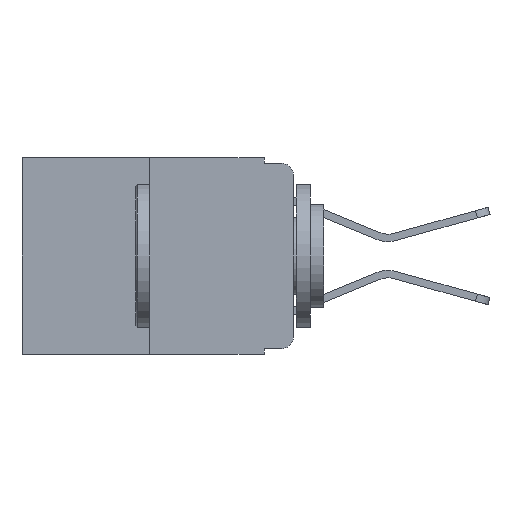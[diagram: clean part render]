
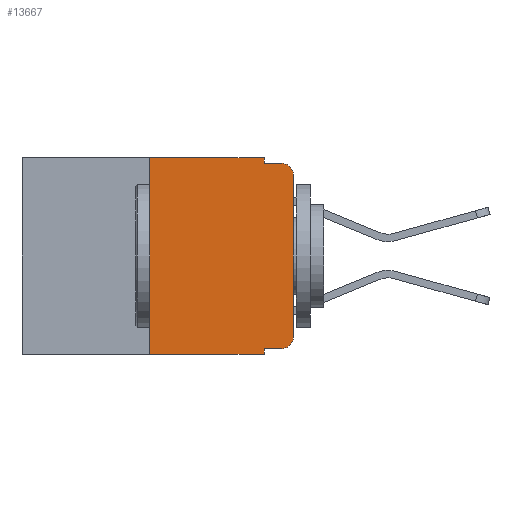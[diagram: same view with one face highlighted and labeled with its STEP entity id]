
A CAD part, left-side view. The second image highlights one B-rep face of the part: STEP entity #13667.
In plain terms, the highlighted planar face has unit normal (-1, 0, 0).
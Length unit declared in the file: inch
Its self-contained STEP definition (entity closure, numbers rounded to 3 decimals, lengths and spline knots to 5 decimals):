
#54 = VERTEX_POINT ( 'NONE', #13120 ) ;
#201 = DIRECTION ( 'NONE',  ( 0., 0., -1. ) ) ;
#498 = CARTESIAN_POINT ( 'NONE',  ( 0., 0.02, -0.333 ) ) ;
#555 = AXIS2_PLACEMENT_3D ( 'NONE', #2039, #13216, #3651 ) ;
#696 = CARTESIAN_POINT ( 'NONE',  ( 0., 0.051, 0. ) ) ;
#766 = CARTESIAN_POINT ( 'NONE',  ( 0., 0., -0.03 ) ) ;
#887 = DIRECTION ( 'NONE',  ( 0., 0., -1. ) ) ;
#2039 = CARTESIAN_POINT ( 'NONE',  ( 0., 0.473, 0. ) ) ;
#2335 = DIRECTION ( 'NONE',  ( 0., -1., 0. ) ) ;
#2366 = DIRECTION ( 'NONE',  ( 0., 0., -1. ) ) ;
#2546 = CARTESIAN_POINT ( 'NONE',  ( 0., 0.25, -0.343 ) ) ;
#2709 = CARTESIAN_POINT ( 'NONE',  ( 0., 0.473, 0. ) ) ;
#3063 = VECTOR ( 'NONE', #2366, 39.37008 ) ;
#3168 = VECTOR ( 'NONE', #6275, 39.37008 ) ;
#3325 = CARTESIAN_POINT ( 'NONE',  ( 0., 0.051, 0. ) ) ;
#3651 = DIRECTION ( 'NONE',  ( 0., 0., -1. ) ) ;
#3678 = ORIENTED_EDGE ( 'NONE', *, *, #8463, .T. ) ;
#3805 = VECTOR ( 'NONE', #9018, 39.37008 ) ;
#3898 = VERTEX_POINT ( 'NONE', #766 ) ;
#4137 = CIRCLE ( 'NONE', #9452, 0.02 ) ;
#4145 = VERTEX_POINT ( 'NONE', #18810 ) ;
#4224 = VERTEX_POINT ( 'NONE', #14356 ) ;
#4323 = LINE ( 'NONE', #2709, #3805 ) ;
#4458 = VERTEX_POINT ( 'NONE', #10040 ) ;
#5120 = VERTEX_POINT ( 'NONE', #498 ) ;
#5843 = EDGE_CURVE ( 'NONE', #19342, #4224, #14138, .T. ) ;
#5881 = EDGE_LOOP ( 'NONE', ( #9590, #20347, #9848, #18756, #19218, #12920, #13413, #7420, #3678, #17368 ) ) ;
#5967 = EDGE_CURVE ( 'NONE', #54, #4224, #19871, .T. ) ;
#6275 = DIRECTION ( 'NONE',  ( 0., 0., -1. ) ) ;
#6377 = EDGE_CURVE ( 'NONE', #5120, #4145, #4137, .T. ) ;
#6899 = AXIS2_PLACEMENT_3D ( 'NONE', #19210, #9796, #201 ) ;
#7038 = EDGE_CURVE ( 'NONE', #19342, #4458, #16535, .T. ) ;
#7420 = ORIENTED_EDGE ( 'NONE', *, *, #5967, .F. ) ;
#7806 = DIRECTION ( 'NONE',  ( 0., 0., 1. ) ) ;
#8083 = VECTOR ( 'NONE', #7806, 39.37008 ) ;
#8146 = VERTEX_POINT ( 'NONE', #16918 ) ;
#8390 = VERTEX_POINT ( 'NONE', #19013 ) ;
#8463 = EDGE_CURVE ( 'NONE', #54, #5120, #17715, .T. ) ;
#8648 = CARTESIAN_POINT ( 'NONE',  ( 0., 0.051, -0.01 ) ) ;
#9018 = DIRECTION ( 'NONE',  ( 0., -1., 0. ) ) ;
#9261 = VECTOR ( 'NONE', #19206, 39.37008 ) ;
#9452 = AXIS2_PLACEMENT_3D ( 'NONE', #19821, #10475, #887 ) ;
#9590 = ORIENTED_EDGE ( 'NONE', *, *, #16605, .T. ) ;
#9796 = DIRECTION ( 'NONE',  ( -1., 0., 0. ) ) ;
#9848 = ORIENTED_EDGE ( 'NONE', *, *, #11305, .F. ) ;
#10040 = CARTESIAN_POINT ( 'NONE',  ( 0., 0.25, 0. ) ) ;
#10198 = EDGE_CURVE ( 'NONE', #15942, #8390, #15741, .T. ) ;
#10475 = DIRECTION ( 'NONE',  ( -1., 0., 0. ) ) ;
#11305 = EDGE_CURVE ( 'NONE', #8390, #8146, #16418, .T. ) ;
#11511 = PLANE ( 'NONE',  #555 ) ;
#11614 = DIRECTION ( 'NONE',  ( 0., 0., 1. ) ) ;
#12189 = VECTOR ( 'NONE', #2335, 39.37008 ) ;
#12253 = CARTESIAN_POINT ( 'NONE',  ( 0., 0.473, -0.343 ) ) ;
#12376 = EDGE_CURVE ( 'NONE', #3898, #8146, #14705, .T. ) ;
#12920 = ORIENTED_EDGE ( 'NONE', *, *, #7038, .F. ) ;
#12975 = CARTESIAN_POINT ( 'NONE',  ( 0., 0.051, -0.333 ) ) ;
#13120 = CARTESIAN_POINT ( 'NONE',  ( 0., 0.051, -0.333 ) ) ;
#13216 = DIRECTION ( 'NONE',  ( 1., 0., 0. ) ) ;
#13413 = ORIENTED_EDGE ( 'NONE', *, *, #5843, .T. ) ;
#13645 = VECTOR ( 'NONE', #18548, 39.37008 ) ;
#13667 = ADVANCED_FACE ( 'NONE', ( #15976 ), #11511, .F. ) ;
#14138 = LINE ( 'NONE', #12253, #13645 ) ;
#14211 = CARTESIAN_POINT ( 'NONE',  ( 0., 0.25, 0. ) ) ;
#14356 = CARTESIAN_POINT ( 'NONE',  ( 0., 0.051, -0.343 ) ) ;
#14705 = CIRCLE ( 'NONE', #6899, 0.02 ) ;
#15033 = VECTOR ( 'NONE', #11614, 39.37008 ) ;
#15741 = LINE ( 'NONE', #696, #3063 ) ;
#15799 = CARTESIAN_POINT ( 'NONE',  ( 0., 0.051, 0. ) ) ;
#15942 = VERTEX_POINT ( 'NONE', #3325 ) ;
#15976 = FACE_OUTER_BOUND ( 'NONE', #5881, .T. ) ;
#16418 = LINE ( 'NONE', #8648, #12189 ) ;
#16535 = LINE ( 'NONE', #14211, #8083 ) ;
#16605 = EDGE_CURVE ( 'NONE', #4145, #3898, #20051, .T. ) ;
#16918 = CARTESIAN_POINT ( 'NONE',  ( 0., 0.02, -0.01 ) ) ;
#17055 = EDGE_CURVE ( 'NONE', #4458, #15942, #4323, .T. ) ;
#17368 = ORIENTED_EDGE ( 'NONE', *, *, #6377, .T. ) ;
#17715 = LINE ( 'NONE', #12975, #9261 ) ;
#18548 = DIRECTION ( 'NONE',  ( 0., -1., 0. ) ) ;
#18756 = ORIENTED_EDGE ( 'NONE', *, *, #10198, .F. ) ;
#18810 = CARTESIAN_POINT ( 'NONE',  ( 0., 0., -0.313 ) ) ;
#19013 = CARTESIAN_POINT ( 'NONE',  ( 0., 0.051, -0.01 ) ) ;
#19206 = DIRECTION ( 'NONE',  ( 0., -1., 0. ) ) ;
#19210 = CARTESIAN_POINT ( 'NONE',  ( 0., 0.02, -0.03 ) ) ;
#19218 = ORIENTED_EDGE ( 'NONE', *, *, #17055, .F. ) ;
#19342 = VERTEX_POINT ( 'NONE', #2546 ) ;
#19393 = CARTESIAN_POINT ( 'NONE',  ( 0., 0., 0. ) ) ;
#19821 = CARTESIAN_POINT ( 'NONE',  ( 0., 0.02, -0.313 ) ) ;
#19871 = LINE ( 'NONE', #15799, #3168 ) ;
#20051 = LINE ( 'NONE', #19393, #15033 ) ;
#20347 = ORIENTED_EDGE ( 'NONE', *, *, #12376, .T. ) ;
